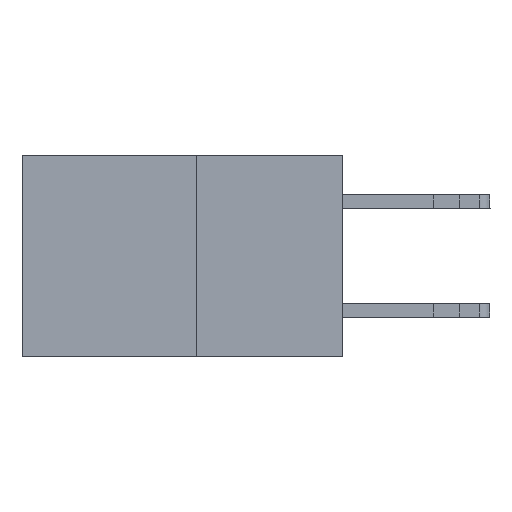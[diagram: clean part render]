
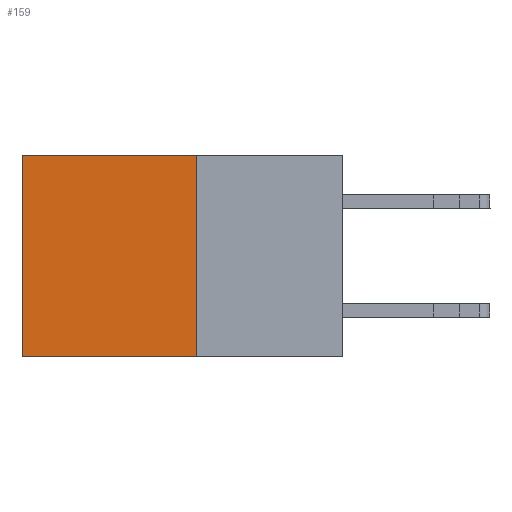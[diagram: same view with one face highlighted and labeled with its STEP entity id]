
A CAD part, left-side view. The second image highlights one B-rep face of the part: STEP entity #159.
In plain terms, the highlighted planar face has unit normal (-1, 0, 0).
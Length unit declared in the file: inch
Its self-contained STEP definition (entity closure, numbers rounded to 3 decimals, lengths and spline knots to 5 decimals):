
#51 = CARTESIAN_POINT ( 'NONE',  ( 0.277, 0.59, 0. ) ) ;
#159 = ADVANCED_FACE ( 'NONE', ( #14667 ), #12449, .F. ) ;
#270 = CARTESIAN_POINT ( 'NONE',  ( 0.277, 0.27, 0. ) ) ;
#333 = CARTESIAN_POINT ( 'NONE',  ( 0.277, 0.59, -0.37 ) ) ;
#383 = CARTESIAN_POINT ( 'NONE',  ( 0.277, 0.27, -0.37 ) ) ;
#889 = LINE ( 'NONE', #383, #11758 ) ;
#1100 = VECTOR ( 'NONE', #16630, 39.37008 ) ;
#2005 = ORIENTED_EDGE ( 'NONE', *, *, #16485, .F. ) ;
#2630 = CARTESIAN_POINT ( 'NONE',  ( 0.277, 0.59, -0.37 ) ) ;
#3544 = LINE ( 'NONE', #8764, #13922 ) ;
#4076 = VERTEX_POINT ( 'NONE', #270 ) ;
#4768 = VERTEX_POINT ( 'NONE', #10211 ) ;
#5369 = CARTESIAN_POINT ( 'NONE',  ( 0.277, 0.27, -0.37 ) ) ;
#5676 = AXIS2_PLACEMENT_3D ( 'NONE', #11356, #12515, #12773 ) ;
#6063 = EDGE_CURVE ( 'NONE', #16828, #7924, #6065, .T. ) ;
#6065 = LINE ( 'NONE', #333, #12676 ) ;
#7543 = EDGE_LOOP ( 'NONE', ( #13393, #14093, #2005, #10149 ) ) ;
#7811 = DIRECTION ( 'NONE',  ( 0., 0., -1. ) ) ;
#7924 = VERTEX_POINT ( 'NONE', #2630 ) ;
#8764 = CARTESIAN_POINT ( 'NONE',  ( 0.277, 0.27, 0. ) ) ;
#10149 = ORIENTED_EDGE ( 'NONE', *, *, #17961, .T. ) ;
#10211 = CARTESIAN_POINT ( 'NONE',  ( 0.277, 0.27, -0.37 ) ) ;
#10285 = DIRECTION ( 'NONE',  ( 0., 0., -1. ) ) ;
#11356 = CARTESIAN_POINT ( 'NONE',  ( 0.277, 0.27, -0.37 ) ) ;
#11758 = VECTOR ( 'NONE', #7811, 39.37008 ) ;
#12449 = PLANE ( 'NONE',  #5676 ) ;
#12515 = DIRECTION ( 'NONE',  ( 1., 0., 0. ) ) ;
#12676 = VECTOR ( 'NONE', #10285, 39.37008 ) ;
#12773 = DIRECTION ( 'NONE',  ( 0., 0., -1. ) ) ;
#13393 = ORIENTED_EDGE ( 'NONE', *, *, #6063, .T. ) ;
#13922 = VECTOR ( 'NONE', #17184, 39.37008 ) ;
#14093 = ORIENTED_EDGE ( 'NONE', *, *, #16677, .F. ) ;
#14667 = FACE_OUTER_BOUND ( 'NONE', #7543, .T. ) ;
#16144 = LINE ( 'NONE', #5369, #1100 ) ;
#16485 = EDGE_CURVE ( 'NONE', #4076, #4768, #889, .T. ) ;
#16630 = DIRECTION ( 'NONE',  ( 0., 1., 0. ) ) ;
#16677 = EDGE_CURVE ( 'NONE', #4768, #7924, #16144, .T. ) ;
#16828 = VERTEX_POINT ( 'NONE', #51 ) ;
#17184 = DIRECTION ( 'NONE',  ( 0., 1., 0. ) ) ;
#17961 = EDGE_CURVE ( 'NONE', #4076, #16828, #3544, .T. ) ;
